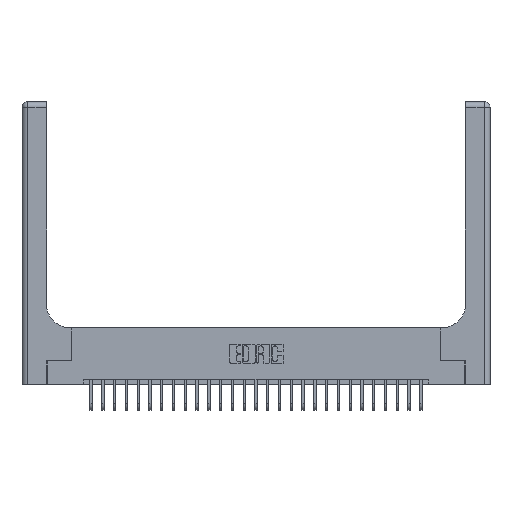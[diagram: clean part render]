
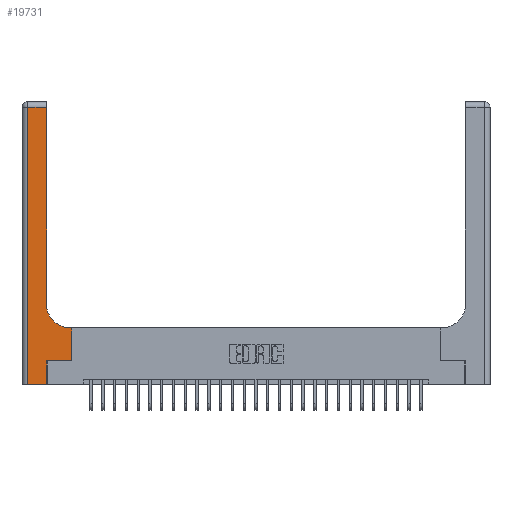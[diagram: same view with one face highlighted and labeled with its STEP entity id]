
A CAD part, top view. The second image highlights one B-rep face of the part: STEP entity #19731.
In plain terms, the highlighted planar face has unit normal (0, 0, 1).
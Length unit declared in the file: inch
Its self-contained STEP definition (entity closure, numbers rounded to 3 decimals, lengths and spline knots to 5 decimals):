
#762 = LINE ( 'NONE', #9416, #8172 ) ;
#1033 = ORIENTED_EDGE ( 'NONE', *, *, #12076, .T. ) ;
#1237 = VECTOR ( 'NONE', #13393, 39.37008 ) ;
#1378 = LINE ( 'NONE', #18739, #3529 ) ;
#1705 = ORIENTED_EDGE ( 'NONE', *, *, #10073, .T. ) ;
#1819 = VECTOR ( 'NONE', #1878, 39.37008 ) ;
#1878 = DIRECTION ( 'NONE',  ( 0., -1., 0. ) ) ;
#2956 = EDGE_CURVE ( 'NONE', #12604, #5333, #9568, .T. ) ;
#3263 = VERTEX_POINT ( 'NONE', #9817 ) ;
#3529 = VECTOR ( 'NONE', #7921, 39.37008 ) ;
#5333 = VERTEX_POINT ( 'NONE', #8648 ) ;
#7134 = CARTESIAN_POINT ( 'NONE',  ( 0., 2.94, 0.37 ) ) ;
#7365 = VERTEX_POINT ( 'NONE', #7727 ) ;
#7727 = CARTESIAN_POINT ( 'NONE',  ( 0.528, 0.6, 0.37 ) ) ;
#7921 = DIRECTION ( 'NONE',  ( -1., 0., 0. ) ) ;
#8172 = VECTOR ( 'NONE', #18105, 39.37008 ) ;
#8648 = CARTESIAN_POINT ( 'NONE',  ( 0.26, 2.94, 0.37 ) ) ;
#8752 = DIRECTION ( 'NONE',  ( 0., 1., 0. ) ) ;
#8955 = ORIENTED_EDGE ( 'NONE', *, *, #17590, .T. ) ;
#8970 = VECTOR ( 'NONE', #12633, 39.37008 ) ;
#9265 = DIRECTION ( 'NONE',  ( 1., 0., 0. ) ) ;
#9416 = CARTESIAN_POINT ( 'NONE',  ( 0., 0., 0.37 ) ) ;
#9568 = LINE ( 'NONE', #18254, #13815 ) ;
#9817 = CARTESIAN_POINT ( 'NONE',  ( 0.06, 0., 0.37 ) ) ;
#10073 = EDGE_CURVE ( 'NONE', #25390, #19356, #11680, .T. ) ;
#10176 = ORIENTED_EDGE ( 'NONE', *, *, #24994, .T. ) ;
#10269 = VECTOR ( 'NONE', #9265, 39.37008 ) ;
#10597 = CARTESIAN_POINT ( 'NONE',  ( 0.265, 0., 0.37 ) ) ;
#10649 = DIRECTION ( 'NONE',  ( 0., 0., -1. ) ) ;
#11557 = EDGE_CURVE ( 'NONE', #19356, #7365, #23033, .T. ) ;
#11680 = LINE ( 'NONE', #20092, #10269 ) ;
#12076 = EDGE_CURVE ( 'NONE', #7365, #27233, #1378, .T. ) ;
#12604 = VERTEX_POINT ( 'NONE', #23530 ) ;
#12633 = DIRECTION ( 'NONE',  ( 0., 1., 0. ) ) ;
#13203 = PLANE ( 'NONE',  #19048 ) ;
#13257 = LINE ( 'NONE', #7134, #1237 ) ;
#13393 = DIRECTION ( 'NONE',  ( -1., 0., 0. ) ) ;
#13653 = CARTESIAN_POINT ( 'NONE',  ( 0.51, 0.6, 0.37 ) ) ;
#13815 = VECTOR ( 'NONE', #24807, 39.37008 ) ;
#14107 = CARTESIAN_POINT ( 'NONE',  ( 0.06, 2.94, 0.37 ) ) ;
#14335 = EDGE_CURVE ( 'NONE', #27773, #3263, #15388, .T. ) ;
#15162 = LINE ( 'NONE', #10597, #27347 ) ;
#15250 = DIRECTION ( 'NONE',  ( 0., 0., -1. ) ) ;
#15254 = VERTEX_POINT ( 'NONE', #22517 ) ;
#15276 = CARTESIAN_POINT ( 'NONE',  ( 0.265, 0.25, 0.37 ) ) ;
#15388 = LINE ( 'NONE', #23782, #1819 ) ;
#15515 = CARTESIAN_POINT ( 'NONE',  ( 0.528, 0.25, 0.37 ) ) ;
#16346 = AXIS2_PLACEMENT_3D ( 'NONE', #25489, #15250, #23923 ) ;
#16475 = ORIENTED_EDGE ( 'NONE', *, *, #21104, .T. ) ;
#16476 = ORIENTED_EDGE ( 'NONE', *, *, #20853, .T. ) ;
#17590 = EDGE_CURVE ( 'NONE', #5333, #27773, #13257, .T. ) ;
#18007 = ORIENTED_EDGE ( 'NONE', *, *, #11557, .T. ) ;
#18105 = DIRECTION ( 'NONE',  ( 1., 0., 0. ) ) ;
#18254 = CARTESIAN_POINT ( 'NONE',  ( 0.26, 3., 0.37 ) ) ;
#18739 = CARTESIAN_POINT ( 'NONE',  ( 0.26, 0.6, 0.37 ) ) ;
#19048 = AXIS2_PLACEMENT_3D ( 'NONE', #25882, #10649, #21884 ) ;
#19356 = VERTEX_POINT ( 'NONE', #15515 ) ;
#19731 = ADVANCED_FACE ( 'NONE', ( #24021 ), #13203, .F. ) ;
#20092 = CARTESIAN_POINT ( 'NONE',  ( 0.265, 0.25, 0.37 ) ) ;
#20816 = EDGE_LOOP ( 'NONE', ( #22910, #8955, #27948, #16476, #10176, #1705, #18007, #1033, #16475 ) ) ;
#20853 = EDGE_CURVE ( 'NONE', #3263, #15254, #762, .T. ) ;
#21104 = EDGE_CURVE ( 'NONE', #27233, #12604, #24982, .T. ) ;
#21884 = DIRECTION ( 'NONE',  ( -1., 0., 0. ) ) ;
#22517 = CARTESIAN_POINT ( 'NONE',  ( 0.265, 0., 0.37 ) ) ;
#22910 = ORIENTED_EDGE ( 'NONE', *, *, #2956, .T. ) ;
#23033 = LINE ( 'NONE', #23600, #8970 ) ;
#23530 = CARTESIAN_POINT ( 'NONE',  ( 0.26, 0.85, 0.37 ) ) ;
#23600 = CARTESIAN_POINT ( 'NONE',  ( 0.528, 0.25, 0.37 ) ) ;
#23782 = CARTESIAN_POINT ( 'NONE',  ( 0.06, 3., 0.37 ) ) ;
#23923 = DIRECTION ( 'NONE',  ( 1., 0., 0. ) ) ;
#24021 = FACE_OUTER_BOUND ( 'NONE', #20816, .T. ) ;
#24807 = DIRECTION ( 'NONE',  ( 0., 1., 0. ) ) ;
#24982 = CIRCLE ( 'NONE', #16346, 0.25 ) ;
#24994 = EDGE_CURVE ( 'NONE', #15254, #25390, #15162, .T. ) ;
#25390 = VERTEX_POINT ( 'NONE', #15276 ) ;
#25489 = CARTESIAN_POINT ( 'NONE',  ( 0.51, 0.85, 0.37 ) ) ;
#25882 = CARTESIAN_POINT ( 'NONE',  ( 0., 3., 0.37 ) ) ;
#27233 = VERTEX_POINT ( 'NONE', #13653 ) ;
#27347 = VECTOR ( 'NONE', #8752, 39.37008 ) ;
#27773 = VERTEX_POINT ( 'NONE', #14107 ) ;
#27948 = ORIENTED_EDGE ( 'NONE', *, *, #14335, .T. ) ;
